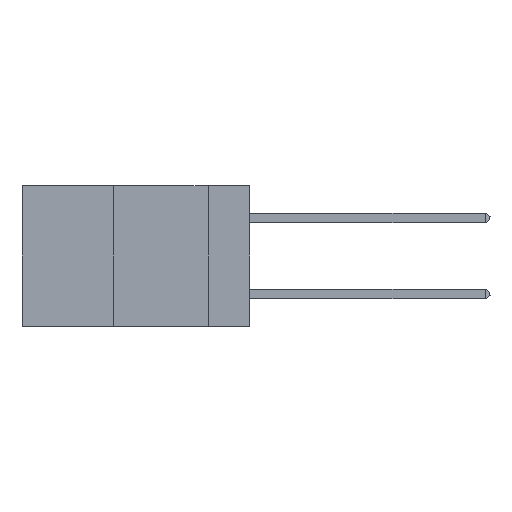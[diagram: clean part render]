
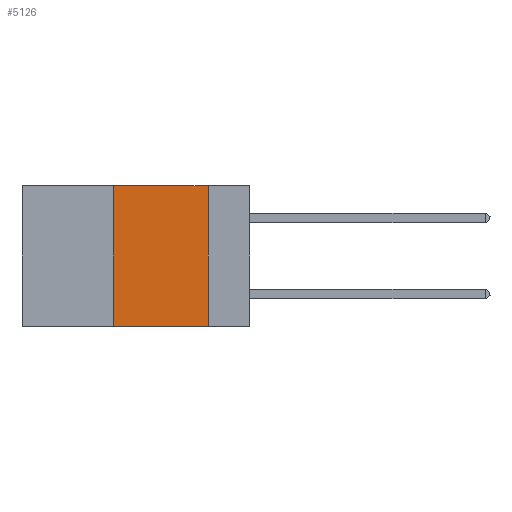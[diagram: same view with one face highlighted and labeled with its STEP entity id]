
A CAD part, left-side view. The second image highlights one B-rep face of the part: STEP entity #5126.
In plain terms, the highlighted planar face has unit normal (-1, 0, 0).
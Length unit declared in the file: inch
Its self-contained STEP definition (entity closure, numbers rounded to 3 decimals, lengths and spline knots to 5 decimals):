
#298 = LINE ( 'NONE', #10857, #24080 ) ;
#394 = EDGE_CURVE ( 'NONE', #24893, #3414, #15545, .T. ) ;
#1410 = CARTESIAN_POINT ( 'NONE',  ( 0., 0.11, -0.37 ) ) ;
#3414 = VERTEX_POINT ( 'NONE', #24369 ) ;
#3839 = AXIS2_PLACEMENT_3D ( 'NONE', #6505, #25671, #27985 ) ;
#3929 = PLANE ( 'NONE',  #3839 ) ;
#5126 = ADVANCED_FACE ( 'NONE', ( #5911 ), #3929, .F. ) ;
#5865 = EDGE_CURVE ( 'NONE', #23121, #23020, #24975, .T. ) ;
#5911 = FACE_OUTER_BOUND ( 'NONE', #17474, .T. ) ;
#6505 = CARTESIAN_POINT ( 'NONE',  ( 0., 0.6, 0. ) ) ;
#7937 = CARTESIAN_POINT ( 'NONE',  ( 0., 0.36, -0.37 ) ) ;
#8892 = CARTESIAN_POINT ( 'NONE',  ( 0., 0.36, 0. ) ) ;
#9431 = VECTOR ( 'NONE', #20558, 39.37008 ) ;
#10857 = CARTESIAN_POINT ( 'NONE',  ( 0., 0.6, 0. ) ) ;
#11688 = ORIENTED_EDGE ( 'NONE', *, *, #5865, .F. ) ;
#12454 = LINE ( 'NONE', #29092, #24780 ) ;
#12965 = DIRECTION ( 'NONE',  ( 0., -1., 0. ) ) ;
#15545 = LINE ( 'NONE', #8892, #9431 ) ;
#15665 = EDGE_CURVE ( 'NONE', #24893, #23020, #12454, .T. ) ;
#15688 = DIRECTION ( 'NONE',  ( 0., 0., -1. ) ) ;
#17474 = EDGE_LOOP ( 'NONE', ( #11688, #17594, #25245, #27586 ) ) ;
#17594 = ORIENTED_EDGE ( 'NONE', *, *, #22916, .F. ) ;
#18482 = VECTOR ( 'NONE', #15688, 39.37008 ) ;
#20558 = DIRECTION ( 'NONE',  ( 0., 0., 1. ) ) ;
#20765 = DIRECTION ( 'NONE',  ( 0., -1., 0. ) ) ;
#22916 = EDGE_CURVE ( 'NONE', #3414, #23121, #298, .T. ) ;
#23020 = VERTEX_POINT ( 'NONE', #1410 ) ;
#23121 = VERTEX_POINT ( 'NONE', #24910 ) ;
#24080 = VECTOR ( 'NONE', #12965, 39.37008 ) ;
#24369 = CARTESIAN_POINT ( 'NONE',  ( 0., 0.36, 0. ) ) ;
#24780 = VECTOR ( 'NONE', #20765, 39.37008 ) ;
#24893 = VERTEX_POINT ( 'NONE', #7937 ) ;
#24910 = CARTESIAN_POINT ( 'NONE',  ( 0., 0.11, 0. ) ) ;
#24975 = LINE ( 'NONE', #29442, #18482 ) ;
#25245 = ORIENTED_EDGE ( 'NONE', *, *, #394, .F. ) ;
#25671 = DIRECTION ( 'NONE',  ( 1., 0., 0. ) ) ;
#27586 = ORIENTED_EDGE ( 'NONE', *, *, #15665, .T. ) ;
#27985 = DIRECTION ( 'NONE',  ( 0., 0., -1. ) ) ;
#29092 = CARTESIAN_POINT ( 'NONE',  ( 0., 0.6, -0.37 ) ) ;
#29442 = CARTESIAN_POINT ( 'NONE',  ( 0., 0.11, 0. ) ) ;
